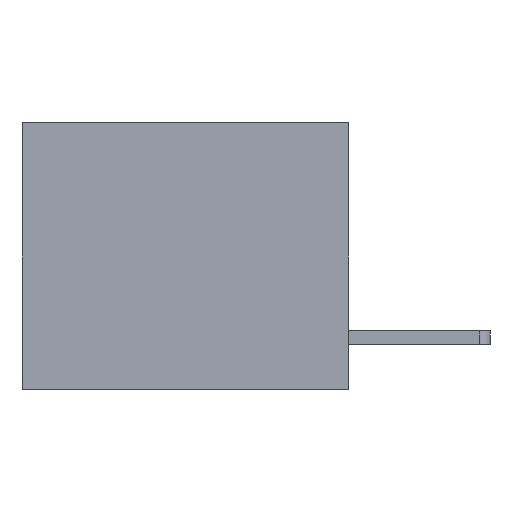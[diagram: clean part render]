
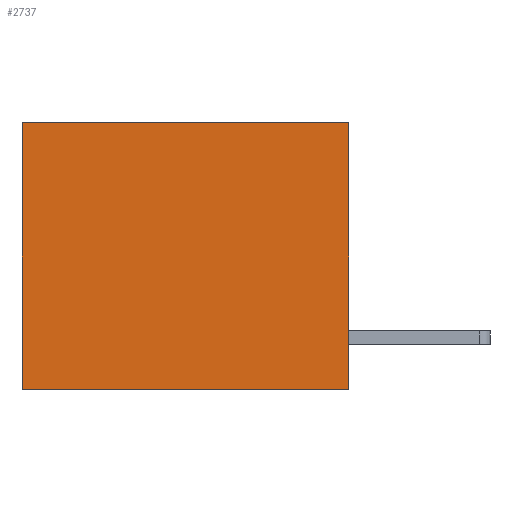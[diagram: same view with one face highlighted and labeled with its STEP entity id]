
A CAD part, left-side view. The second image highlights one B-rep face of the part: STEP entity #2737.
In plain terms, the highlighted planar face has unit normal (-1, 0, 0).
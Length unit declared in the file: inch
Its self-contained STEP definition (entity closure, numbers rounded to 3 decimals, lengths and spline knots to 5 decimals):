
#576 = CARTESIAN_POINT ( 'NONE',  ( 0.3165, 0., 0. ) ) ;
#1935 = VECTOR ( 'NONE', #8482, 39.37008 ) ;
#1976 = CARTESIAN_POINT ( 'NONE',  ( 0.3165, 0., -0.49 ) ) ;
#2061 = CARTESIAN_POINT ( 'NONE',  ( 0.3165, 0.6, -0.49 ) ) ;
#2120 = VERTEX_POINT ( 'NONE', #7657 ) ;
#2171 = EDGE_CURVE ( 'NONE', #3919, #8808, #3105, .T. ) ;
#2737 = ADVANCED_FACE ( 'NONE', ( #3227 ), #5015, .F. ) ;
#2939 = LINE ( 'NONE', #1976, #1935 ) ;
#3061 = CARTESIAN_POINT ( 'NONE',  ( 0.3165, 0., 0. ) ) ;
#3105 = LINE ( 'NONE', #4102, #7869 ) ;
#3216 = VECTOR ( 'NONE', #11243, 39.37008 ) ;
#3227 = FACE_OUTER_BOUND ( 'NONE', #9630, .T. ) ;
#3353 = ORIENTED_EDGE ( 'NONE', *, *, #2171, .F. ) ;
#3797 = LINE ( 'NONE', #2061, #3216 ) ;
#3919 = VERTEX_POINT ( 'NONE', #8580 ) ;
#4102 = CARTESIAN_POINT ( 'NONE',  ( 0.3165, 0., -0.49 ) ) ;
#4121 = CARTESIAN_POINT ( 'NONE',  ( 0.3165, 0., -0.49 ) ) ;
#4335 = VECTOR ( 'NONE', #8856, 39.37008 ) ;
#4532 = VERTEX_POINT ( 'NONE', #3061 ) ;
#5015 = PLANE ( 'NONE',  #5971 ) ;
#5903 = DIRECTION ( 'NONE',  ( 1., 0., 0. ) ) ;
#5971 = AXIS2_PLACEMENT_3D ( 'NONE', #4121, #5903, #11406 ) ;
#6761 = DIRECTION ( 'NONE',  ( 0., 1., 0. ) ) ;
#6782 = LINE ( 'NONE', #576, #4335 ) ;
#7116 = EDGE_CURVE ( 'NONE', #4532, #3919, #2939, .T. ) ;
#7126 = EDGE_CURVE ( 'NONE', #2120, #8808, #3797, .T. ) ;
#7657 = CARTESIAN_POINT ( 'NONE',  ( 0.3165, 0.6, 0. ) ) ;
#7718 = CARTESIAN_POINT ( 'NONE',  ( 0.3165, 0.6, -0.49 ) ) ;
#7869 = VECTOR ( 'NONE', #6761, 39.37008 ) ;
#8482 = DIRECTION ( 'NONE',  ( 0., 0., -1. ) ) ;
#8580 = CARTESIAN_POINT ( 'NONE',  ( 0.3165, 0., -0.49 ) ) ;
#8782 = ORIENTED_EDGE ( 'NONE', *, *, #8876, .T. ) ;
#8808 = VERTEX_POINT ( 'NONE', #7718 ) ;
#8856 = DIRECTION ( 'NONE',  ( 0., 1., 0. ) ) ;
#8876 = EDGE_CURVE ( 'NONE', #4532, #2120, #6782, .T. ) ;
#8953 = ORIENTED_EDGE ( 'NONE', *, *, #7116, .F. ) ;
#9630 = EDGE_LOOP ( 'NONE', ( #9970, #3353, #8953, #8782 ) ) ;
#9970 = ORIENTED_EDGE ( 'NONE', *, *, #7126, .T. ) ;
#11243 = DIRECTION ( 'NONE',  ( 0., 0., -1. ) ) ;
#11406 = DIRECTION ( 'NONE',  ( 0., 0., -1. ) ) ;
